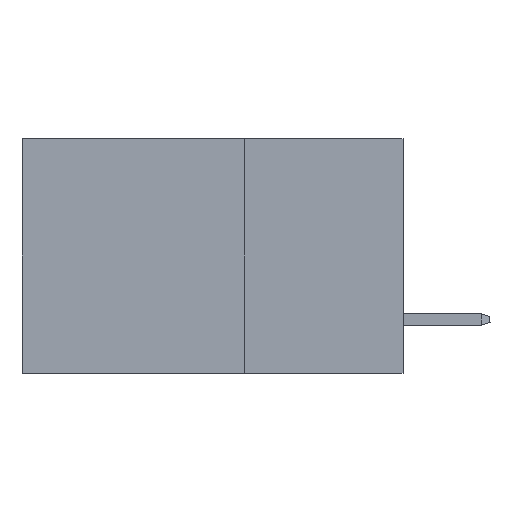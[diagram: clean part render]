
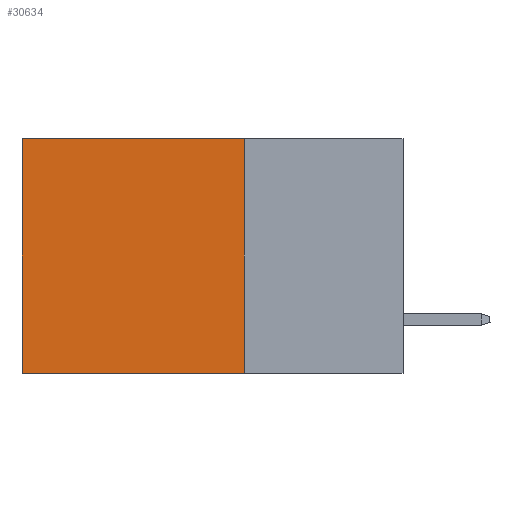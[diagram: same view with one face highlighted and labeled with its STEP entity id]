
A CAD part, left-side view. The second image highlights one B-rep face of the part: STEP entity #30634.
In plain terms, the highlighted planar face has unit normal (-1, 0, 0).
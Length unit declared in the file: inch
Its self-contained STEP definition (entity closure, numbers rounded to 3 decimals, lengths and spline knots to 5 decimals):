
#598 = EDGE_CURVE ( 'NONE', #23351, #20358, #15579, .T. ) ;
#909 = DIRECTION ( 'NONE',  ( 0., 1., 0. ) ) ;
#1115 = CARTESIAN_POINT ( 'NONE',  ( 0.2875, 0.25, 0. ) ) ;
#2806 = ORIENTED_EDGE ( 'NONE', *, *, #598, .T. ) ;
#4464 = EDGE_CURVE ( 'NONE', #23351, #17605, #27489, .T. ) ;
#5237 = DIRECTION ( 'NONE',  ( 0., 0., -1. ) ) ;
#5797 = FACE_OUTER_BOUND ( 'NONE', #7898, .T. ) ;
#6777 = VECTOR ( 'NONE', #33629, 39.37008 ) ;
#7157 = CARTESIAN_POINT ( 'NONE',  ( 0.2875, 0.25, 0. ) ) ;
#7757 = CARTESIAN_POINT ( 'NONE',  ( 0.2875, 0.25, -0.37 ) ) ;
#7898 = EDGE_LOOP ( 'NONE', ( #25660, #35850, #21021, #2806 ) ) ;
#8603 = EDGE_CURVE ( 'NONE', #20358, #14306, #32300, .T. ) ;
#11941 = PLANE ( 'NONE',  #18796 ) ;
#12496 = CARTESIAN_POINT ( 'NONE',  ( 0.2875, 0.25, 0. ) ) ;
#14306 = VERTEX_POINT ( 'NONE', #34229 ) ;
#15579 = LINE ( 'NONE', #1115, #29378 ) ;
#15933 = LINE ( 'NONE', #31516, #31511 ) ;
#17605 = VERTEX_POINT ( 'NONE', #7757 ) ;
#18796 = AXIS2_PLACEMENT_3D ( 'NONE', #27131, #38837, #39027 ) ;
#20358 = VERTEX_POINT ( 'NONE', #38873 ) ;
#21021 = ORIENTED_EDGE ( 'NONE', *, *, #4464, .F. ) ;
#23248 = CARTESIAN_POINT ( 'NONE',  ( 0.2875, 0.6, 0. ) ) ;
#23351 = VERTEX_POINT ( 'NONE', #7157 ) ;
#25660 = ORIENTED_EDGE ( 'NONE', *, *, #8603, .T. ) ;
#27131 = CARTESIAN_POINT ( 'NONE',  ( 0.2875, 0.25, 0. ) ) ;
#27489 = LINE ( 'NONE', #12496, #6777 ) ;
#29057 = EDGE_CURVE ( 'NONE', #17605, #14306, #15933, .T. ) ;
#29378 = VECTOR ( 'NONE', #909, 39.37008 ) ;
#30634 = ADVANCED_FACE ( 'NONE', ( #5797 ), #11941, .F. ) ;
#31511 = VECTOR ( 'NONE', #34088, 39.37008 ) ;
#31516 = CARTESIAN_POINT ( 'NONE',  ( 0.2875, 0.25, -0.37 ) ) ;
#32300 = LINE ( 'NONE', #23248, #35393 ) ;
#33629 = DIRECTION ( 'NONE',  ( 0., 0., -1. ) ) ;
#34088 = DIRECTION ( 'NONE',  ( 0., 1., 0. ) ) ;
#34229 = CARTESIAN_POINT ( 'NONE',  ( 0.2875, 0.6, -0.37 ) ) ;
#35393 = VECTOR ( 'NONE', #5237, 39.37008 ) ;
#35850 = ORIENTED_EDGE ( 'NONE', *, *, #29057, .F. ) ;
#38837 = DIRECTION ( 'NONE',  ( 1., 0., 0. ) ) ;
#38873 = CARTESIAN_POINT ( 'NONE',  ( 0.2875, 0.6, 0. ) ) ;
#39027 = DIRECTION ( 'NONE',  ( 0., 0., -1. ) ) ;
